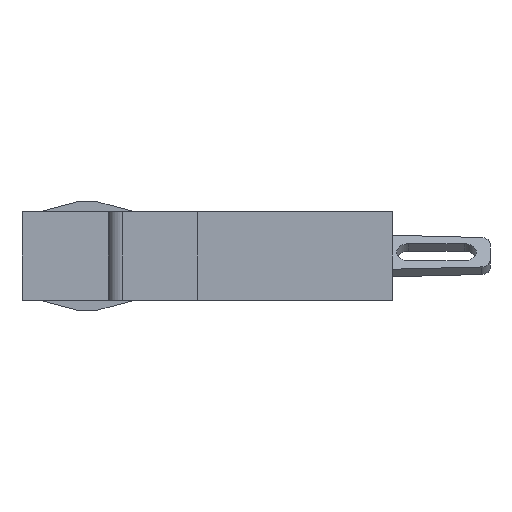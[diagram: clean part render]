
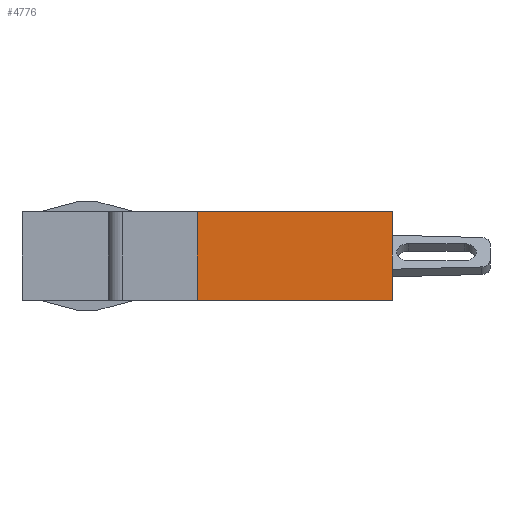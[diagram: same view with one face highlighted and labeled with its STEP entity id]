
A CAD part, left-side view. The second image highlights one B-rep face of the part: STEP entity #4776.
In plain terms, the highlighted planar face has unit normal (-1, 0, 0).
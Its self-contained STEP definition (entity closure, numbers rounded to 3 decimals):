
#18 = CARTESIAN_POINT ( 'NONE',  ( -2.235, -11.176, -2.54 ) ) ;
#41 = DIRECTION ( 'NONE',  ( 0., 1., 0. ) ) ;
#439 = FACE_OUTER_BOUND ( 'NONE', #2993, .T. ) ;
#591 = VECTOR ( 'NONE', #3691, 1000. ) ;
#708 = CARTESIAN_POINT ( 'NONE',  ( -2.235, -11.176, 2.54 ) ) ;
#1567 = ORIENTED_EDGE ( 'NONE', *, *, #5489, .T. ) ;
#1627 = EDGE_CURVE ( 'NONE', #4241, #5661, #1882, .T. ) ;
#1685 = ORIENTED_EDGE ( 'NONE', *, *, #5242, .T. ) ;
#1882 = LINE ( 'NONE', #708, #3054 ) ;
#1895 = ORIENTED_EDGE ( 'NONE', *, *, #5140, .F. ) ;
#2106 = DIRECTION ( 'NONE',  ( 0., 0., 1. ) ) ;
#2256 = VECTOR ( 'NONE', #2106, 1000. ) ;
#2399 = AXIS2_PLACEMENT_3D ( 'NONE', #4469, #6564, #6035 ) ;
#2993 = EDGE_LOOP ( 'NONE', ( #5500, #1685, #1895, #1567 ) ) ;
#3054 = VECTOR ( 'NONE', #6517, 1000. ) ;
#3473 = PLANE ( 'NONE',  #2399 ) ;
#3691 = DIRECTION ( 'NONE',  ( 0., 0., -1. ) ) ;
#3748 = LINE ( 'NONE', #4775, #5222 ) ;
#4241 = VERTEX_POINT ( 'NONE', #4247 ) ;
#4247 = CARTESIAN_POINT ( 'NONE',  ( -2.235, -11.176, 2.54 ) ) ;
#4264 = CARTESIAN_POINT ( 'NONE',  ( -2.235, 0., 2.54 ) ) ;
#4469 = CARTESIAN_POINT ( 'NONE',  ( -2.235, -11.176, -2.54 ) ) ;
#4775 = CARTESIAN_POINT ( 'NONE',  ( -2.235, -11.176, -2.54 ) ) ;
#4776 = ADVANCED_FACE ( 'NONE', ( #439 ), #3473, .T. ) ;
#4819 = CARTESIAN_POINT ( 'NONE',  ( -2.235, 0., 2.54 ) ) ;
#5060 = LINE ( 'NONE', #18, #2256 ) ;
#5140 = EDGE_CURVE ( 'NONE', #6586, #5577, #3748, .T. ) ;
#5222 = VECTOR ( 'NONE', #41, 1000. ) ;
#5242 = EDGE_CURVE ( 'NONE', #5661, #5577, #5900, .T. ) ;
#5489 = EDGE_CURVE ( 'NONE', #6586, #4241, #5060, .T. ) ;
#5500 = ORIENTED_EDGE ( 'NONE', *, *, #1627, .T. ) ;
#5577 = VERTEX_POINT ( 'NONE', #6642 ) ;
#5661 = VERTEX_POINT ( 'NONE', #4819 ) ;
#5843 = CARTESIAN_POINT ( 'NONE',  ( -2.235, -11.176, -2.54 ) ) ;
#5900 = LINE ( 'NONE', #4264, #591 ) ;
#6035 = DIRECTION ( 'NONE',  ( 0., 0., 1. ) ) ;
#6517 = DIRECTION ( 'NONE',  ( 0., 1., 0. ) ) ;
#6564 = DIRECTION ( 'NONE',  ( -1., 0., 0. ) ) ;
#6586 = VERTEX_POINT ( 'NONE', #5843 ) ;
#6642 = CARTESIAN_POINT ( 'NONE',  ( -2.235, 0., -2.54 ) ) ;
